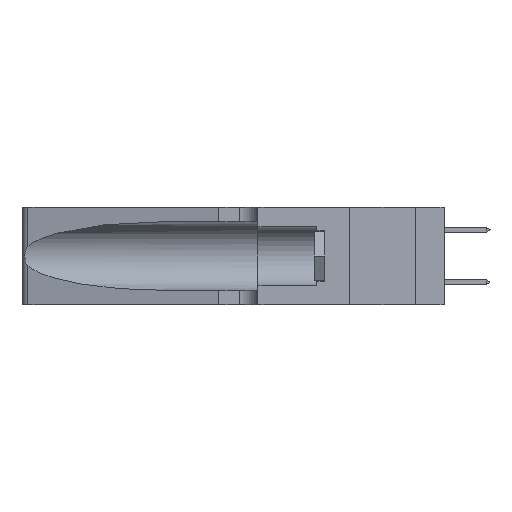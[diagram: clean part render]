
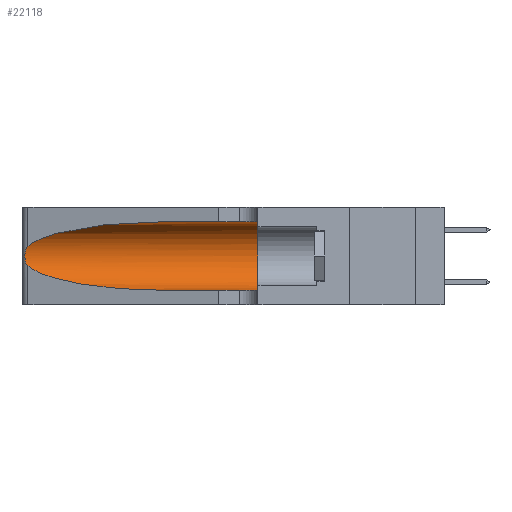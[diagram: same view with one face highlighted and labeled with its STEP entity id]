
A CAD part, left-side view. The second image highlights one B-rep face of the part: STEP entity #22118.
In plain terms, the highlighted cylindrical face has radius 3.308 mm (diameter 6.617 mm), a partial arc.
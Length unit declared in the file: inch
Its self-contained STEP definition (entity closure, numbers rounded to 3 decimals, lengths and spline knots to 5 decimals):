
#1030 = CARTESIAN_POINT ( 'NONE',  ( 0.1305, 1.61858, 0.185 ) ) ;
#1156 = CARTESIAN_POINT ( 'NONE',  ( 0.1305, 0.72297, 0.31525 ) ) ;
#1242 = CARTESIAN_POINT ( 'NONE',  ( 0.26075, 1.23896, 0.19203 ) ) ;
#1766 = LINE ( 'NONE', #16114, #10860 ) ;
#2947 = FACE_OUTER_BOUND ( 'NONE', #11564, .T. ) ;
#3224 = CARTESIAN_POINT ( 'NONE',  ( 0.26017, 1.23833, 0.17102 ) ) ;
#3460 = CARTESIAN_POINT ( 'NONE',  ( 0.1305, 0.72297, 0.31525 ) ) ;
#4141 = VERTEX_POINT ( 'NONE', #3460 ) ;
#4174 = VECTOR ( 'NONE', #6797, 39.37008 ) ;
#5050 = CARTESIAN_POINT ( 'NONE',  ( 0.2373, 1.15595, 0.28018 ) ) ;
#5053 = CARTESIAN_POINT ( 'NONE',  ( 0.25555, 1.22994, 0.2215 ) ) ;
#5144 = CARTESIAN_POINT ( 'NONE',  ( 0.25789, 1.23486, 0.15765 ) ) ;
#6302 = CARTESIAN_POINT ( 'NONE',  ( 0.25487, 1.22718, 0.14631 ) ) ;
#6530 = VERTEX_POINT ( 'NONE', #21717 ) ;
#6797 = DIRECTION ( 'NONE',  ( 0., -1., 0. ) ) ;
#6869 = ORIENTED_EDGE ( 'NONE', *, *, #21307, .F. ) ;
#6870 = DIRECTION ( 'NONE',  ( 0., 0., -1. ) ) ;
#7090 = CARTESIAN_POINT ( 'NONE',  ( 0.25555, 1.22993, 0.14849 ) ) ;
#7300 = ORIENTED_EDGE ( 'NONE', *, *, #17935, .T. ) ;
#7900 = EDGE_CURVE ( 'NONE', #19690, #21836, #20140, .T. ) ;
#8107 =( BOUNDED_CURVE ( )  B_SPLINE_CURVE ( 3, ( #6302, #17837, #19771, #8256 ),
 .UNSPECIFIED., .F., .F. ) 
 B_SPLINE_CURVE_WITH_KNOTS ( ( 4, 4 ),
 ( 3.44316, 4.71239 ),
 .UNSPECIFIED. ) 
 CURVE ( )  GEOMETRIC_REPRESENTATION_ITEM ( )  RATIONAL_B_SPLINE_CURVE ( ( 1., 0.87, 0.87, 1. ) ) 
 REPRESENTATION_ITEM ( '' )  );
#8253 = CIRCLE ( 'NONE', #16335, 0.13025 ) ;
#8256 = CARTESIAN_POINT ( 'NONE',  ( 0.1305, 0.72297, 0.05475 ) ) ;
#8392 = ORIENTED_EDGE ( 'NONE', *, *, #7900, .T. ) ;
#9808 = DIRECTION ( 'NONE',  ( 0., 1., 0. ) ) ;
#10017 = AXIS2_PLACEMENT_3D ( 'NONE', #1030, #18396, #6870 ) ;
#10413 = CARTESIAN_POINT ( 'NONE',  ( 0.25487, 1.22718, 0.14631 ) ) ;
#10860 = VECTOR ( 'NONE', #19952, 39.37008 ) ;
#10912 = CARTESIAN_POINT ( 'NONE',  ( 0.25787, 1.23484, 0.2124 ) ) ;
#11150 = VERTEX_POINT ( 'NONE', #10413 ) ;
#11564 = EDGE_LOOP ( 'NONE', ( #7300, #13067, #24629, #8392, #14814, #6869 ) ) ;
#11610 = EDGE_CURVE ( 'NONE', #6530, #21836, #8253, .T. ) ;
#11678 = CARTESIAN_POINT ( 'NONE',  ( 0.25487, 1.22718, 0.22369 ) ) ;
#12602 =( BOUNDED_CURVE ( )  B_SPLINE_CURVE ( 3, ( #1156, #16608, #5050, #18522 ),
 .UNSPECIFIED., .F., .T. ) 
 B_SPLINE_CURVE_WITH_KNOTS ( ( 4, 4 ),
 ( 1.5708, 2.84003 ),
 .UNSPECIFIED. ) 
 CURVE ( )  GEOMETRIC_REPRESENTATION_ITEM ( )  RATIONAL_B_SPLINE_CURVE ( ( 1., 0.87, 0.87, 1. ) ) 
 REPRESENTATION_ITEM ( '' )  );
#12763 = CARTESIAN_POINT ( 'NONE',  ( 0.25487, 1.22718, 0.22369 ) ) ;
#12844 = CARTESIAN_POINT ( 'NONE',  ( 0.26018, 1.23835, 0.19895 ) ) ;
#13067 = ORIENTED_EDGE ( 'NONE', *, *, #19799, .T. ) ;
#14433 = CARTESIAN_POINT ( 'NONE',  ( 0.1305, 0.72297, 0.05475 ) ) ;
#14768 = CARTESIAN_POINT ( 'NONE',  ( 0.26075, 1.23896, 0.178 ) ) ;
#14814 = ORIENTED_EDGE ( 'NONE', *, *, #11610, .F. ) ;
#16114 = CARTESIAN_POINT ( 'NONE',  ( 0.1305, 1.61858, 0.31525 ) ) ;
#16335 = AXIS2_PLACEMENT_3D ( 'NONE', #21300, #9808, #23230 ) ;
#16608 = CARTESIAN_POINT ( 'NONE',  ( 0.18966, 0.96281, 0.31525 ) ) ;
#16684 = CARTESIAN_POINT ( 'NONE',  ( 0.25856, 1.23593, 0.16098 ) ) ;
#17545 = VERTEX_POINT ( 'NONE', #11678 ) ;
#17837 = CARTESIAN_POINT ( 'NONE',  ( 0.2373, 1.15595, 0.08982 ) ) ;
#17935 = EDGE_CURVE ( 'NONE', #4141, #17545, #12602, .T. ) ;
#18351 = EDGE_CURVE ( 'NONE', #11150, #19690, #8107, .T. ) ;
#18396 = DIRECTION ( 'NONE',  ( 0., -1., 0. ) ) ;
#18522 = CARTESIAN_POINT ( 'NONE',  ( 0.25487, 1.22718, 0.22369 ) ) ;
#18614 = CARTESIAN_POINT ( 'NONE',  ( 0.25639, 1.23186, 0.15144 ) ) ;
#19690 = VERTEX_POINT ( 'NONE', #14433 ) ;
#19771 = CARTESIAN_POINT ( 'NONE',  ( 0.18966, 0.96281, 0.05475 ) ) ;
#19799 = EDGE_CURVE ( 'NONE', #17545, #11150, #24136, .T. ) ;
#19952 = DIRECTION ( 'NONE',  ( 0., -1., 0. ) ) ;
#20140 = LINE ( 'NONE', #24057, #4174 ) ;
#20563 = CARTESIAN_POINT ( 'NONE',  ( 0.25487, 1.22718, 0.14631 ) ) ;
#21300 = CARTESIAN_POINT ( 'NONE',  ( 0.1305, 0.35, 0.185 ) ) ;
#21307 = EDGE_CURVE ( 'NONE', #4141, #6530, #1766, .T. ) ;
#21717 = CARTESIAN_POINT ( 'NONE',  ( 0.1305, 0.35, 0.31525 ) ) ;
#21836 = VERTEX_POINT ( 'NONE', #23379 ) ;
#22118 = ADVANCED_FACE ( 'NONE', ( #2947 ), #22212, .F. ) ;
#22212 = CYLINDRICAL_SURFACE ( 'NONE', #10017, 0.13025 ) ;
#22396 = CARTESIAN_POINT ( 'NONE',  ( 0.25639, 1.23184, 0.21858 ) ) ;
#23230 = DIRECTION ( 'NONE',  ( 0., 0., 1. ) ) ;
#23379 = CARTESIAN_POINT ( 'NONE',  ( 0.1305, 0.35, 0.05475 ) ) ;
#24057 = CARTESIAN_POINT ( 'NONE',  ( 0.1305, 1.61858, 0.05475 ) ) ;
#24136 = B_SPLINE_CURVE_WITH_KNOTS ( 'NONE', 3,
 ( #12763, #5053, #22396, #10912, #24346, #12844, #1242, #14768, #3224, #16684, #5144, #18614, #7090, #20563 ),
 .UNSPECIFIED., .F., .F.,
 ( 4, 2, 2, 2, 2, 2, 4 ),
 ( 0., 0.00027, 0.00053, 0.00107, 0.0016, 0.00187, 0.00214 ),
 .UNSPECIFIED. ) ;
#24346 = CARTESIAN_POINT ( 'NONE',  ( 0.25854, 1.2359, 0.20912 ) ) ;
#24629 = ORIENTED_EDGE ( 'NONE', *, *, #18351, .T. ) ;
